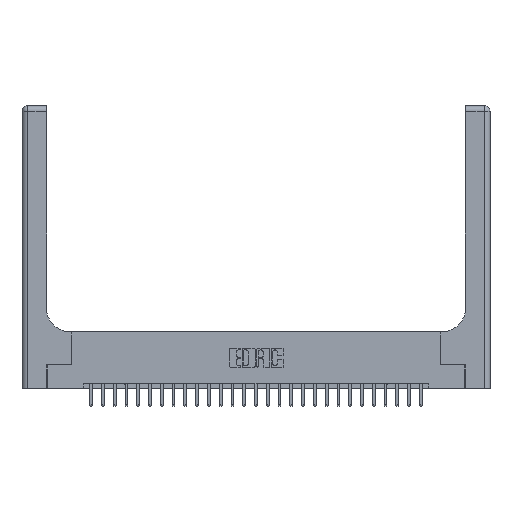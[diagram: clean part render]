
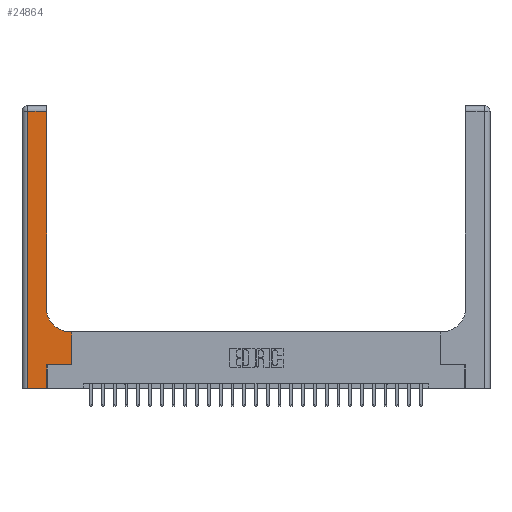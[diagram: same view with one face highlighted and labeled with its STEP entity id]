
A CAD part, top view. The second image highlights one B-rep face of the part: STEP entity #24864.
In plain terms, the highlighted planar face has unit normal (0, 0, 1).
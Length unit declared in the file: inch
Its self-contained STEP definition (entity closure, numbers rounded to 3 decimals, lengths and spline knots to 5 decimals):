
#794 = VERTEX_POINT ( 'NONE', #9238 ) ;
#1164 = EDGE_LOOP ( 'NONE', ( #3052, #12313, #17366, #12647, #8063, #22728, #1856, #1768, #22523 ) ) ;
#1179 = LINE ( 'NONE', #24139, #25638 ) ;
#1662 = VECTOR ( 'NONE', #12076, 39.37008 ) ;
#1741 = CARTESIAN_POINT ( 'NONE',  ( 0.51, 0.85, 0.37 ) ) ;
#1752 = LINE ( 'NONE', #5893, #23730 ) ;
#1768 = ORIENTED_EDGE ( 'NONE', *, *, #20384, .T. ) ;
#1781 = CARTESIAN_POINT ( 'NONE',  ( 0.528, 0.25, 0.37 ) ) ;
#1818 = CARTESIAN_POINT ( 'NONE',  ( 0.26, 0.6, 0.37 ) ) ;
#1856 = ORIENTED_EDGE ( 'NONE', *, *, #5579, .T. ) ;
#2248 = DIRECTION ( 'NONE',  ( 0., 1., 0. ) ) ;
#2615 = LINE ( 'NONE', #24143, #1662 ) ;
#2674 = VECTOR ( 'NONE', #23837, 39.37008 ) ;
#3052 = ORIENTED_EDGE ( 'NONE', *, *, #7001, .T. ) ;
#3610 = CIRCLE ( 'NONE', #19869, 0.25 ) ;
#3749 = VECTOR ( 'NONE', #16398, 39.37008 ) ;
#4083 = EDGE_CURVE ( 'NONE', #794, #21350, #6254, .T. ) ;
#4855 = CARTESIAN_POINT ( 'NONE',  ( 0.51, 0.6, 0.37 ) ) ;
#5553 = DIRECTION ( 'NONE',  ( -1., 0., 0. ) ) ;
#5579 = EDGE_CURVE ( 'NONE', #12469, #13131, #15668, .T. ) ;
#5893 = CARTESIAN_POINT ( 'NONE',  ( 0.06, 3., 0.37 ) ) ;
#6254 = LINE ( 'NONE', #14380, #3749 ) ;
#7001 = EDGE_CURVE ( 'NONE', #17667, #794, #1179, .T. ) ;
#7323 = DIRECTION ( 'NONE',  ( 0., 0., -1. ) ) ;
#7937 = VERTEX_POINT ( 'NONE', #17247 ) ;
#8063 = ORIENTED_EDGE ( 'NONE', *, *, #18383, .T. ) ;
#9238 = CARTESIAN_POINT ( 'NONE',  ( 0.26, 2.94, 0.37 ) ) ;
#9307 = AXIS2_PLACEMENT_3D ( 'NONE', #19254, #7323, #5553 ) ;
#10018 = DIRECTION ( 'NONE',  ( 0., 0., -1. ) ) ;
#10661 = VECTOR ( 'NONE', #23448, 39.37008 ) ;
#10904 = LINE ( 'NONE', #1818, #15616 ) ;
#12011 = DIRECTION ( 'NONE',  ( 0., 1., 0. ) ) ;
#12076 = DIRECTION ( 'NONE',  ( 1., 0., 0. ) ) ;
#12313 = ORIENTED_EDGE ( 'NONE', *, *, #4083, .T. ) ;
#12469 = VERTEX_POINT ( 'NONE', #12714 ) ;
#12647 = ORIENTED_EDGE ( 'NONE', *, *, #16948, .T. ) ;
#12706 = CARTESIAN_POINT ( 'NONE',  ( 0.06, 0., 0.37 ) ) ;
#12714 = CARTESIAN_POINT ( 'NONE',  ( 0.528, 0.25, 0.37 ) ) ;
#13116 = CARTESIAN_POINT ( 'NONE',  ( 0.06, 2.94, 0.37 ) ) ;
#13131 = VERTEX_POINT ( 'NONE', #23003 ) ;
#14085 = CARTESIAN_POINT ( 'NONE',  ( 0., 0., 0.37 ) ) ;
#14380 = CARTESIAN_POINT ( 'NONE',  ( 0., 2.94, 0.37 ) ) ;
#14734 = FACE_OUTER_BOUND ( 'NONE', #1164, .T. ) ;
#15232 = CARTESIAN_POINT ( 'NONE',  ( 0.26, 0.85, 0.37 ) ) ;
#15536 = LINE ( 'NONE', #25497, #17721 ) ;
#15616 = VECTOR ( 'NONE', #25738, 39.37008 ) ;
#15668 = LINE ( 'NONE', #1781, #10661 ) ;
#15982 = VERTEX_POINT ( 'NONE', #4855 ) ;
#16398 = DIRECTION ( 'NONE',  ( -1., 0., 0. ) ) ;
#16948 = EDGE_CURVE ( 'NONE', #24602, #24279, #22757, .T. ) ;
#17247 = CARTESIAN_POINT ( 'NONE',  ( 0.265, 0.25, 0.37 ) ) ;
#17366 = ORIENTED_EDGE ( 'NONE', *, *, #19673, .T. ) ;
#17667 = VERTEX_POINT ( 'NONE', #15232 ) ;
#17721 = VECTOR ( 'NONE', #12011, 39.37008 ) ;
#18383 = EDGE_CURVE ( 'NONE', #24279, #7937, #15536, .T. ) ;
#19254 = CARTESIAN_POINT ( 'NONE',  ( 0., 3., 0.37 ) ) ;
#19521 = CARTESIAN_POINT ( 'NONE',  ( 0.265, 0., 0.37 ) ) ;
#19673 = EDGE_CURVE ( 'NONE', #21350, #24602, #1752, .T. ) ;
#19869 = AXIS2_PLACEMENT_3D ( 'NONE', #1741, #10018, #25925 ) ;
#20384 = EDGE_CURVE ( 'NONE', #13131, #15982, #10904, .T. ) ;
#21350 = VERTEX_POINT ( 'NONE', #13116 ) ;
#22249 = EDGE_CURVE ( 'NONE', #7937, #12469, #2615, .T. ) ;
#22523 = ORIENTED_EDGE ( 'NONE', *, *, #25715, .T. ) ;
#22728 = ORIENTED_EDGE ( 'NONE', *, *, #22249, .T. ) ;
#22757 = LINE ( 'NONE', #14085, #2674 ) ;
#23003 = CARTESIAN_POINT ( 'NONE',  ( 0.528, 0.6, 0.37 ) ) ;
#23448 = DIRECTION ( 'NONE',  ( 0., 1., 0. ) ) ;
#23730 = VECTOR ( 'NONE', #24025, 39.37008 ) ;
#23837 = DIRECTION ( 'NONE',  ( 1., 0., 0. ) ) ;
#24025 = DIRECTION ( 'NONE',  ( 0., -1., 0. ) ) ;
#24139 = CARTESIAN_POINT ( 'NONE',  ( 0.26, 3., 0.37 ) ) ;
#24143 = CARTESIAN_POINT ( 'NONE',  ( 0.265, 0.25, 0.37 ) ) ;
#24279 = VERTEX_POINT ( 'NONE', #19521 ) ;
#24602 = VERTEX_POINT ( 'NONE', #12706 ) ;
#24864 = ADVANCED_FACE ( 'NONE', ( #14734 ), #25444, .F. ) ;
#25444 = PLANE ( 'NONE',  #9307 ) ;
#25497 = CARTESIAN_POINT ( 'NONE',  ( 0.265, 0., 0.37 ) ) ;
#25638 = VECTOR ( 'NONE', #2248, 39.37008 ) ;
#25715 = EDGE_CURVE ( 'NONE', #15982, #17667, #3610, .T. ) ;
#25738 = DIRECTION ( 'NONE',  ( -1., 0., 0. ) ) ;
#25925 = DIRECTION ( 'NONE',  ( 1., 0., 0. ) ) ;
